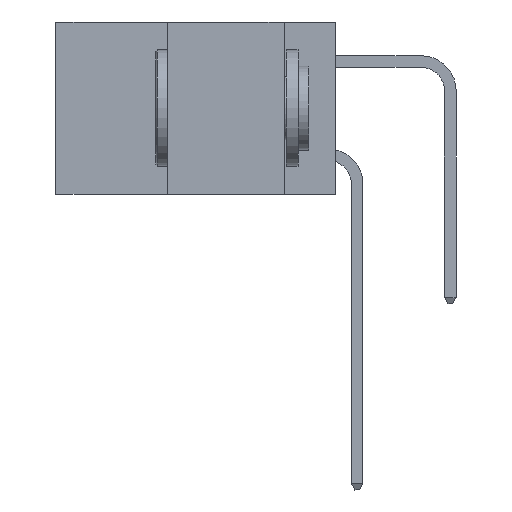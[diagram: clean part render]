
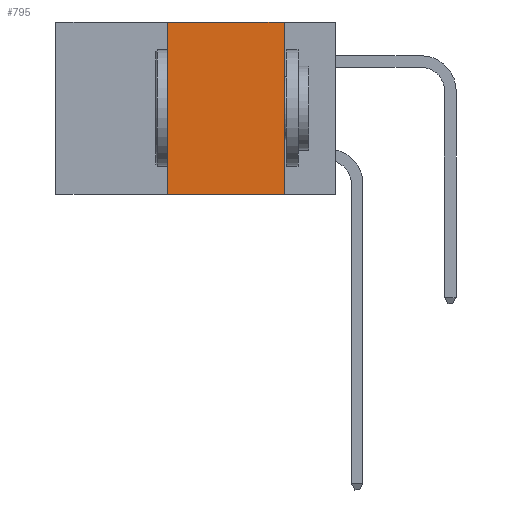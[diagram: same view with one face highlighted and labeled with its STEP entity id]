
A CAD part, left-side view. The second image highlights one B-rep face of the part: STEP entity #795.
In plain terms, the highlighted planar face has unit normal (-1, 0, 0).
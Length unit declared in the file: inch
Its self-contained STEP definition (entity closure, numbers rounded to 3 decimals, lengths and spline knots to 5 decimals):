
#281 = LINE ( 'NONE', #2849, #4001 ) ;
#795 = ADVANCED_FACE ( 'NONE', ( #8004 ), #11463, .F. ) ;
#810 = VECTOR ( 'NONE', #7830, 39.37008 ) ;
#1458 = CARTESIAN_POINT ( 'NONE',  ( 0., 0.36, 0. ) ) ;
#1496 = CARTESIAN_POINT ( 'NONE',  ( 0., 0.36, 0. ) ) ;
#1765 = LINE ( 'NONE', #9310, #8833 ) ;
#1953 = CARTESIAN_POINT ( 'NONE',  ( 0., 0.11, 0. ) ) ;
#2573 = CARTESIAN_POINT ( 'NONE',  ( 0., 0.11, -0.37 ) ) ;
#2643 = EDGE_CURVE ( 'NONE', #4785, #4819, #1765, .T. ) ;
#2849 = CARTESIAN_POINT ( 'NONE',  ( 0., 0.6, -0.37 ) ) ;
#3865 = EDGE_LOOP ( 'NONE', ( #4266, #11909, #7715, #10569 ) ) ;
#3995 = VERTEX_POINT ( 'NONE', #2573 ) ;
#4001 = VECTOR ( 'NONE', #6362, 39.37008 ) ;
#4057 = CARTESIAN_POINT ( 'NONE',  ( 0., 0.6, 0. ) ) ;
#4266 = ORIENTED_EDGE ( 'NONE', *, *, #11656, .F. ) ;
#4785 = VERTEX_POINT ( 'NONE', #1458 ) ;
#4819 = VERTEX_POINT ( 'NONE', #11092 ) ;
#5055 = DIRECTION ( 'NONE',  ( 0., 0., -1. ) ) ;
#6362 = DIRECTION ( 'NONE',  ( 0., -1., 0. ) ) ;
#6583 = DIRECTION ( 'NONE',  ( 0., -1., 0. ) ) ;
#6597 = VERTEX_POINT ( 'NONE', #7378 ) ;
#6790 = DIRECTION ( 'NONE',  ( 1., 0., 0. ) ) ;
#6986 = AXIS2_PLACEMENT_3D ( 'NONE', #4057, #6790, #5055 ) ;
#7378 = CARTESIAN_POINT ( 'NONE',  ( 0., 0.36, -0.37 ) ) ;
#7715 = ORIENTED_EDGE ( 'NONE', *, *, #8900, .F. ) ;
#7771 = VECTOR ( 'NONE', #7989, 39.37008 ) ;
#7830 = DIRECTION ( 'NONE',  ( 0., 0., -1. ) ) ;
#7989 = DIRECTION ( 'NONE',  ( 0., 0., 1. ) ) ;
#8004 = FACE_OUTER_BOUND ( 'NONE', #3865, .T. ) ;
#8646 = LINE ( 'NONE', #1496, #7771 ) ;
#8833 = VECTOR ( 'NONE', #6583, 39.37008 ) ;
#8900 = EDGE_CURVE ( 'NONE', #6597, #4785, #8646, .T. ) ;
#9262 = EDGE_CURVE ( 'NONE', #6597, #3995, #281, .T. ) ;
#9310 = CARTESIAN_POINT ( 'NONE',  ( 0., 0.6, 0. ) ) ;
#10569 = ORIENTED_EDGE ( 'NONE', *, *, #9262, .T. ) ;
#11092 = CARTESIAN_POINT ( 'NONE',  ( 0., 0.11, 0. ) ) ;
#11220 = LINE ( 'NONE', #1953, #810 ) ;
#11463 = PLANE ( 'NONE',  #6986 ) ;
#11656 = EDGE_CURVE ( 'NONE', #4819, #3995, #11220, .T. ) ;
#11909 = ORIENTED_EDGE ( 'NONE', *, *, #2643, .F. ) ;
